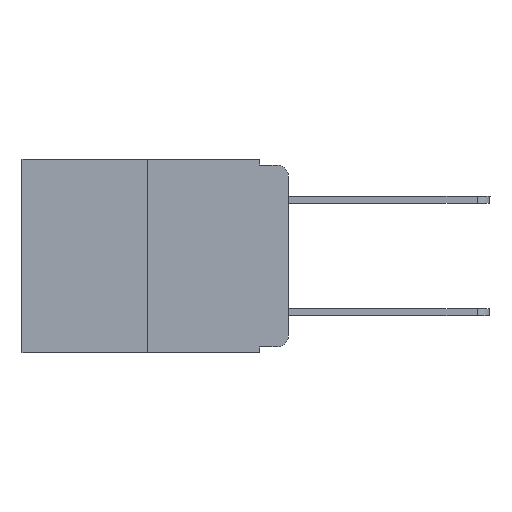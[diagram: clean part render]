
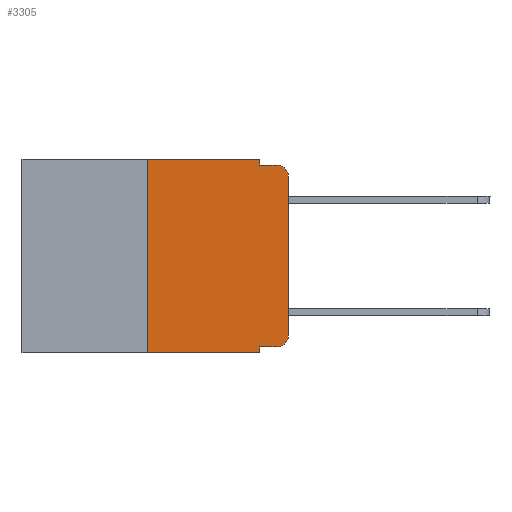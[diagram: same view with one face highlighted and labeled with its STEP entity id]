
A CAD part, left-side view. The second image highlights one B-rep face of the part: STEP entity #3305.
In plain terms, the highlighted planar face has unit normal (-1, 0, 0).
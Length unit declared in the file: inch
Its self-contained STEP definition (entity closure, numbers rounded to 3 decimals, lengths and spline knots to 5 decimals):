
#27 = LINE ( 'NONE', #2220, #9052 ) ;
#70 = VECTOR ( 'NONE', #4978, 39.37008 ) ;
#141 = EDGE_CURVE ( 'NONE', #3397, #20903, #9220, .T. ) ;
#827 = CARTESIAN_POINT ( 'NONE',  ( 0., 0.02, -0.313 ) ) ;
#939 = ORIENTED_EDGE ( 'NONE', *, *, #141, .F. ) ;
#1016 = CARTESIAN_POINT ( 'NONE',  ( 0., 0.02, -0.01 ) ) ;
#1119 = CARTESIAN_POINT ( 'NONE',  ( 0., 0.051, -0.01 ) ) ;
#1585 = PLANE ( 'NONE',  #6461 ) ;
#1688 = EDGE_CURVE ( 'NONE', #14163, #3397, #7019, .T. ) ;
#1733 = ORIENTED_EDGE ( 'NONE', *, *, #10673, .T. ) ;
#1863 = LINE ( 'NONE', #11185, #11509 ) ;
#2199 = CARTESIAN_POINT ( 'NONE',  ( 0., 0.25, 0. ) ) ;
#2220 = CARTESIAN_POINT ( 'NONE',  ( 0., 0.051, -0.333 ) ) ;
#2252 = ORIENTED_EDGE ( 'NONE', *, *, #16144, .F. ) ;
#2736 = EDGE_CURVE ( 'NONE', #16418, #3659, #27, .T. ) ;
#2991 = DIRECTION ( 'NONE',  ( -1., 0., 0. ) ) ;
#3037 = VERTEX_POINT ( 'NONE', #1016 ) ;
#3305 = ADVANCED_FACE ( 'NONE', ( #12606 ), #1585, .F. ) ;
#3397 = VERTEX_POINT ( 'NONE', #2199 ) ;
#3620 = CARTESIAN_POINT ( 'NONE',  ( 0., 0.051, 0. ) ) ;
#3659 = VERTEX_POINT ( 'NONE', #9474 ) ;
#4170 = ORIENTED_EDGE ( 'NONE', *, *, #1688, .F. ) ;
#4284 = ORIENTED_EDGE ( 'NONE', *, *, #19163, .F. ) ;
#4360 = DIRECTION ( 'NONE',  ( 0., 0., -1. ) ) ;
#4978 = DIRECTION ( 'NONE',  ( 0., -1., 0. ) ) ;
#4994 = DIRECTION ( 'NONE',  ( 0., 0., 1. ) ) ;
#5202 = CARTESIAN_POINT ( 'NONE',  ( 0., 0.25, 0. ) ) ;
#6461 = AXIS2_PLACEMENT_3D ( 'NONE', #8967, #23792, #4360 ) ;
#6613 = DIRECTION ( 'NONE',  ( -1., 0., 0. ) ) ;
#7019 = LINE ( 'NONE', #5202, #8201 ) ;
#7939 = VECTOR ( 'NONE', #10672, 39.37008 ) ;
#8084 = CARTESIAN_POINT ( 'NONE',  ( 0., 0.051, 0. ) ) ;
#8199 = LINE ( 'NONE', #8084, #8679 ) ;
#8201 = VECTOR ( 'NONE', #20024, 39.37008 ) ;
#8679 = VECTOR ( 'NONE', #22798, 39.37008 ) ;
#8967 = CARTESIAN_POINT ( 'NONE',  ( 0., 0.473, 0. ) ) ;
#9052 = VECTOR ( 'NONE', #16990, 39.37008 ) ;
#9220 = LINE ( 'NONE', #22222, #18325 ) ;
#9368 = CIRCLE ( 'NONE', #12835, 0.02 ) ;
#9440 = ORIENTED_EDGE ( 'NONE', *, *, #21533, .T. ) ;
#9474 = CARTESIAN_POINT ( 'NONE',  ( 0., 0.02, -0.333 ) ) ;
#9518 = VECTOR ( 'NONE', #4994, 39.37008 ) ;
#9908 = VERTEX_POINT ( 'NONE', #11678 ) ;
#9957 = CARTESIAN_POINT ( 'NONE',  ( 0., 0.051, -0.333 ) ) ;
#10150 = DIRECTION ( 'NONE',  ( 0., 0., -1. ) ) ;
#10524 = CIRCLE ( 'NONE', #11240, 0.02 ) ;
#10672 = DIRECTION ( 'NONE',  ( 0., 0., -1. ) ) ;
#10673 = EDGE_CURVE ( 'NONE', #3659, #9908, #9368, .T. ) ;
#11069 = DIRECTION ( 'NONE',  ( 0., -1., 0. ) ) ;
#11185 = CARTESIAN_POINT ( 'NONE',  ( 0., 0.473, -0.343 ) ) ;
#11240 = AXIS2_PLACEMENT_3D ( 'NONE', #17527, #2991, #11945 ) ;
#11509 = VECTOR ( 'NONE', #11069, 39.37008 ) ;
#11678 = CARTESIAN_POINT ( 'NONE',  ( 0., 0., -0.313 ) ) ;
#11793 = CARTESIAN_POINT ( 'NONE',  ( 0., 0., -0.03 ) ) ;
#11945 = DIRECTION ( 'NONE',  ( 0., 0., -1. ) ) ;
#12031 = VERTEX_POINT ( 'NONE', #11793 ) ;
#12606 = FACE_OUTER_BOUND ( 'NONE', #22632, .T. ) ;
#12704 = CARTESIAN_POINT ( 'NONE',  ( 0., 0.25, -0.343 ) ) ;
#12835 = AXIS2_PLACEMENT_3D ( 'NONE', #827, #6613, #10150 ) ;
#13854 = VERTEX_POINT ( 'NONE', #18716 ) ;
#14163 = VERTEX_POINT ( 'NONE', #12704 ) ;
#14673 = CARTESIAN_POINT ( 'NONE',  ( 0., 0.051, -0.01 ) ) ;
#14822 = EDGE_CURVE ( 'NONE', #12031, #3037, #10524, .T. ) ;
#16144 = EDGE_CURVE ( 'NONE', #19045, #3037, #17967, .T. ) ;
#16336 = ORIENTED_EDGE ( 'NONE', *, *, #14822, .T. ) ;
#16418 = VERTEX_POINT ( 'NONE', #9957 ) ;
#16990 = DIRECTION ( 'NONE',  ( 0., -1., 0. ) ) ;
#17527 = CARTESIAN_POINT ( 'NONE',  ( 0., 0.02, -0.03 ) ) ;
#17943 = LINE ( 'NONE', #3620, #7939 ) ;
#17967 = LINE ( 'NONE', #14673, #70 ) ;
#17988 = LINE ( 'NONE', #21650, #9518 ) ;
#18218 = EDGE_CURVE ( 'NONE', #20903, #19045, #8199, .T. ) ;
#18325 = VECTOR ( 'NONE', #20405, 39.37008 ) ;
#18716 = CARTESIAN_POINT ( 'NONE',  ( 0., 0.051, -0.343 ) ) ;
#19045 = VERTEX_POINT ( 'NONE', #1119 ) ;
#19163 = EDGE_CURVE ( 'NONE', #16418, #13854, #17943, .T. ) ;
#20024 = DIRECTION ( 'NONE',  ( 0., 0., 1. ) ) ;
#20218 = ORIENTED_EDGE ( 'NONE', *, *, #18218, .F. ) ;
#20405 = DIRECTION ( 'NONE',  ( 0., -1., 0. ) ) ;
#20903 = VERTEX_POINT ( 'NONE', #21433 ) ;
#21322 = ORIENTED_EDGE ( 'NONE', *, *, #22883, .T. ) ;
#21433 = CARTESIAN_POINT ( 'NONE',  ( 0., 0.051, 0. ) ) ;
#21533 = EDGE_CURVE ( 'NONE', #9908, #12031, #17988, .T. ) ;
#21650 = CARTESIAN_POINT ( 'NONE',  ( 0., 0., 0. ) ) ;
#22222 = CARTESIAN_POINT ( 'NONE',  ( 0., 0.473, 0. ) ) ;
#22632 = EDGE_LOOP ( 'NONE', ( #9440, #16336, #2252, #20218, #939, #4170, #21322, #4284, #23683, #1733 ) ) ;
#22798 = DIRECTION ( 'NONE',  ( 0., 0., -1. ) ) ;
#22883 = EDGE_CURVE ( 'NONE', #14163, #13854, #1863, .T. ) ;
#23683 = ORIENTED_EDGE ( 'NONE', *, *, #2736, .T. ) ;
#23792 = DIRECTION ( 'NONE',  ( 1., 0., 0. ) ) ;
